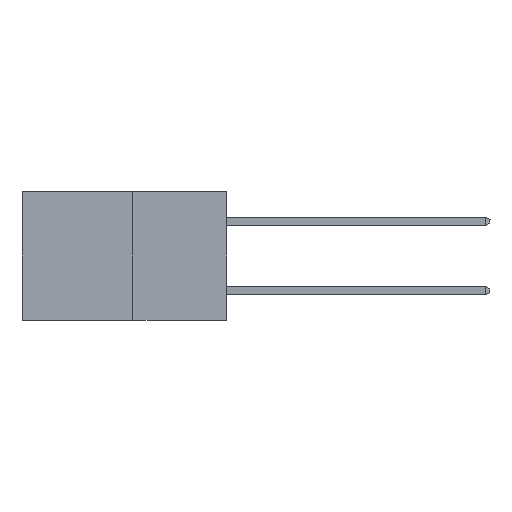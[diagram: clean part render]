
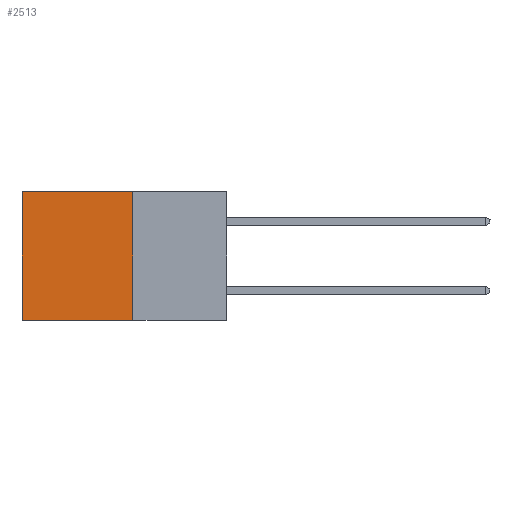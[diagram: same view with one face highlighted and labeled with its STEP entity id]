
A CAD part, left-side view. The second image highlights one B-rep face of the part: STEP entity #2513.
In plain terms, the highlighted planar face has unit normal (-1, 0, 0).
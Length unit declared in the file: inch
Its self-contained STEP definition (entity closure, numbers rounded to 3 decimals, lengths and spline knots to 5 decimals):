
#203 = CARTESIAN_POINT ( 'NONE',  ( 0.277, 0.27, -0.37 ) ) ;
#966 = VERTEX_POINT ( 'NONE', #5282 ) ;
#1464 = CARTESIAN_POINT ( 'NONE',  ( 0.277, 0.27, -0.37 ) ) ;
#1495 = ORIENTED_EDGE ( 'NONE', *, *, #5332, .F. ) ;
#1644 = AXIS2_PLACEMENT_3D ( 'NONE', #1464, #8071, #3570 ) ;
#1674 = EDGE_CURVE ( 'NONE', #5371, #966, #4405, .T. ) ;
#2441 = VECTOR ( 'NONE', #8841, 39.37008 ) ;
#2513 = ADVANCED_FACE ( 'NONE', ( #5702 ), #2567, .F. ) ;
#2567 = PLANE ( 'NONE',  #1644 ) ;
#2918 = DIRECTION ( 'NONE',  ( 0., 0., -1. ) ) ;
#3189 = CARTESIAN_POINT ( 'NONE',  ( 0.277, 0.59, -0.37 ) ) ;
#3322 = LINE ( 'NONE', #6909, #4920 ) ;
#3570 = DIRECTION ( 'NONE',  ( 0., 0., -1. ) ) ;
#4116 = ORIENTED_EDGE ( 'NONE', *, *, #1674, .F. ) ;
#4320 = CARTESIAN_POINT ( 'NONE',  ( 0.277, 0.59, -0.37 ) ) ;
#4330 = LINE ( 'NONE', #8183, #2441 ) ;
#4405 = LINE ( 'NONE', #203, #4611 ) ;
#4429 = CARTESIAN_POINT ( 'NONE',  ( 0.277, 0.59, 0. ) ) ;
#4611 = VECTOR ( 'NONE', #6764, 39.37008 ) ;
#4920 = VECTOR ( 'NONE', #4942, 39.37008 ) ;
#4942 = DIRECTION ( 'NONE',  ( 0., 1., 0. ) ) ;
#4972 = VERTEX_POINT ( 'NONE', #3189 ) ;
#5282 = CARTESIAN_POINT ( 'NONE',  ( 0.277, 0.27, -0.37 ) ) ;
#5332 = EDGE_CURVE ( 'NONE', #966, #4972, #4330, .T. ) ;
#5371 = VERTEX_POINT ( 'NONE', #6890 ) ;
#5702 = FACE_OUTER_BOUND ( 'NONE', #7312, .T. ) ;
#6244 = ORIENTED_EDGE ( 'NONE', *, *, #6292, .T. ) ;
#6245 = VECTOR ( 'NONE', #2918, 39.37008 ) ;
#6292 = EDGE_CURVE ( 'NONE', #5371, #6500, #3322, .T. ) ;
#6356 = EDGE_CURVE ( 'NONE', #6500, #4972, #8045, .T. ) ;
#6500 = VERTEX_POINT ( 'NONE', #4429 ) ;
#6764 = DIRECTION ( 'NONE',  ( 0., 0., -1. ) ) ;
#6890 = CARTESIAN_POINT ( 'NONE',  ( 0.277, 0.27, 0. ) ) ;
#6909 = CARTESIAN_POINT ( 'NONE',  ( 0.277, 0.27, 0. ) ) ;
#7312 = EDGE_LOOP ( 'NONE', ( #7930, #1495, #4116, #6244 ) ) ;
#7930 = ORIENTED_EDGE ( 'NONE', *, *, #6356, .T. ) ;
#8045 = LINE ( 'NONE', #4320, #6245 ) ;
#8071 = DIRECTION ( 'NONE',  ( 1., 0., 0. ) ) ;
#8183 = CARTESIAN_POINT ( 'NONE',  ( 0.277, 0.27, -0.37 ) ) ;
#8841 = DIRECTION ( 'NONE',  ( 0., 1., 0. ) ) ;
